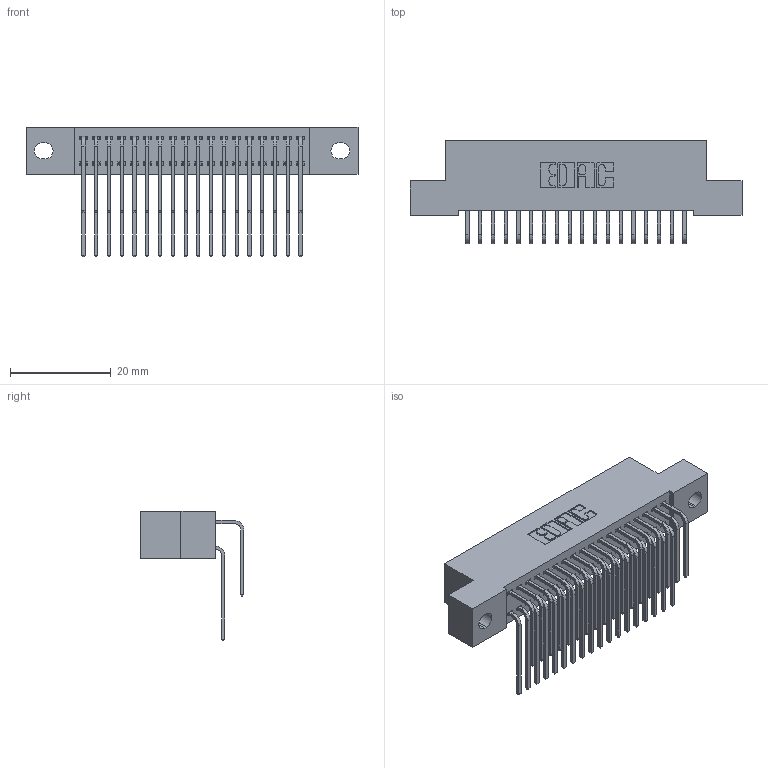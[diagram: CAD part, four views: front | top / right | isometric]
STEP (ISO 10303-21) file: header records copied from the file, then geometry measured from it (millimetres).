
FILE_DESCRIPTION (( 'STEP AP203' ), '1' );
FILE_NAME ('392-036-559-202.STEP', '2018-08-16T04:02:41', ( '' ), ( '' ), 'SwSTEP 2.0', 'SolidWorks 2016', '' );
FILE_SCHEMA (( 'CONFIG_CONTROL_DESIGN' ));
Length unit declared in the file: inch
Products named in the file (4): 342 Part_.128 Slot; 345-292-001_558 559 Tail - 1; 345-292-001_559 Tail - 2; 392-036-559-202
Assembly tree (37 placements, depth 2):
  392-036-559-202
    342 Part_.128 Slot
    345-292-001_558 559 Tail - 1  x18
    345-292-001_559 Tail - 2  x18
Bounding box: 66.04 x 20.64 x 25.78 mm (x, y, z)
Volume: 5975.6 mm3; surface area: 9834.4 mm2
Topology: 37 solids, 37 shells, 2058 faces, 6107 edges, 4022 vertices
Faces by surface type: plane 1438, cylinder 620
Entity records: 16471 total; most frequent: CARTESIAN_POINT 2809, ORIENTED_EDGE 2694, DIRECTION 2423, EDGE_CURVE 1347, LINE 1179, VECTOR 1179, VERTEX_POINT 894, AXIS2_PLACEMENT_3D 622
